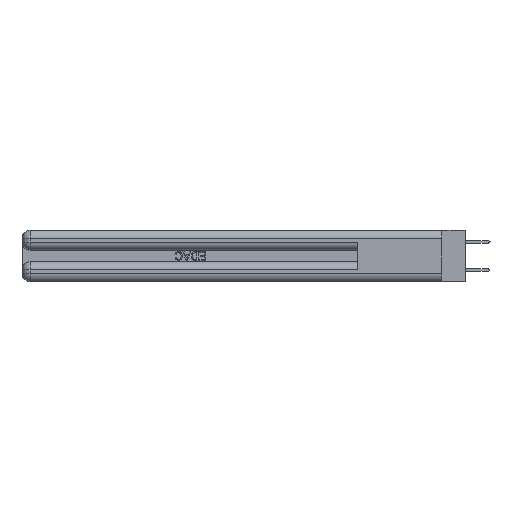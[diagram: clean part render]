
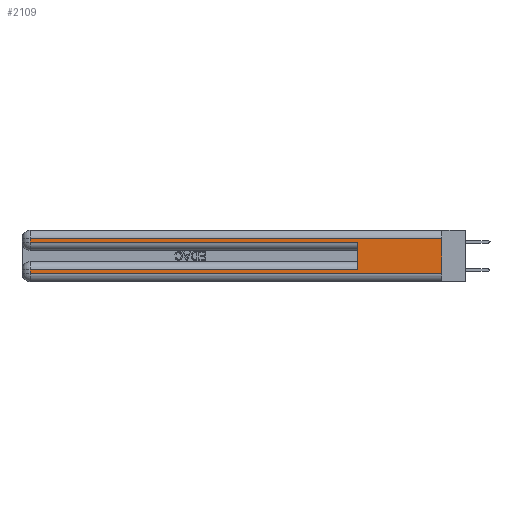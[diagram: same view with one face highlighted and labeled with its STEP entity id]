
A CAD part, left-side view. The second image highlights one B-rep face of the part: STEP entity #2109.
In plain terms, the highlighted planar face has unit normal (-1, 0, 0).
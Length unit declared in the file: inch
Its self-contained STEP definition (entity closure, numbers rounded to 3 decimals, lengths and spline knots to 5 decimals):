
#2109 = ADVANCED_FACE ( 'NONE', ( #13333 ), #38572, .F. ) ;
#3598 = CARTESIAN_POINT ( 'NONE',  ( 0., 0., 0.285 ) ) ;
#4173 = EDGE_CURVE ( 'NONE', #25780, #25477, #43261, .T. ) ;
#4603 = EDGE_CURVE ( 'NONE', #20547, #20723, #4740, .T. ) ;
#4740 = LINE ( 'NONE', #40680, #20423 ) ;
#5199 = LINE ( 'NONE', #25803, #18037 ) ;
#6324 = DIRECTION ( 'NONE',  ( 0., 0., -1. ) ) ;
#6469 = CARTESIAN_POINT ( 'NONE',  ( 0., 2.94, 0.06 ) ) ;
#7218 = VECTOR ( 'NONE', #45504, 39.37008 ) ;
#8037 = DIRECTION ( 'NONE',  ( 0., 1., 0. ) ) ;
#9441 = CARTESIAN_POINT ( 'NONE',  ( 0., 0.6, 0.145 ) ) ;
#11390 = AXIS2_PLACEMENT_3D ( 'NONE', #13796, #22963, #24110 ) ;
#11472 = DIRECTION ( 'NONE',  ( 0., -1., 0. ) ) ;
#12254 = LINE ( 'NONE', #9441, #7218 ) ;
#13333 = FACE_OUTER_BOUND ( 'NONE', #28089, .T. ) ;
#13796 = CARTESIAN_POINT ( 'NONE',  ( 0., 0., 0.37 ) ) ;
#14299 = LINE ( 'NONE', #3598, #29890 ) ;
#14329 = DIRECTION ( 'NONE',  ( 0., -1., 0. ) ) ;
#15424 = CARTESIAN_POINT ( 'NONE',  ( 0., 2.94, 0.285 ) ) ;
#16871 = EDGE_CURVE ( 'NONE', #22562, #25780, #21992, .T. ) ;
#17128 = DIRECTION ( 'NONE',  ( 0., 1., 0. ) ) ;
#17292 = CARTESIAN_POINT ( 'NONE',  ( 0., 0., 0.31 ) ) ;
#18037 = VECTOR ( 'NONE', #11472, 39.37008 ) ;
#19333 = DIRECTION ( 'NONE',  ( 0., 0., -1. ) ) ;
#20137 = CARTESIAN_POINT ( 'NONE',  ( 0., 0.6, 0.085 ) ) ;
#20184 = VERTEX_POINT ( 'NONE', #20137 ) ;
#20280 = ORIENTED_EDGE ( 'NONE', *, *, #42400, .T. ) ;
#20293 = VECTOR ( 'NONE', #17128, 39.37008 ) ;
#20423 = VECTOR ( 'NONE', #19333, 39.37008 ) ;
#20547 = VERTEX_POINT ( 'NONE', #36850 ) ;
#20723 = VERTEX_POINT ( 'NONE', #6469 ) ;
#21463 = VECTOR ( 'NONE', #8037, 39.37008 ) ;
#21992 = LINE ( 'NONE', #42281, #21463 ) ;
#22198 = CARTESIAN_POINT ( 'NONE',  ( 0., 0., 0.37 ) ) ;
#22562 = VERTEX_POINT ( 'NONE', #17292 ) ;
#22963 = DIRECTION ( 'NONE',  ( 1., 0., 0. ) ) ;
#23842 = VERTEX_POINT ( 'NONE', #34713 ) ;
#24110 = DIRECTION ( 'NONE',  ( 0., 0., -1. ) ) ;
#25477 = VERTEX_POINT ( 'NONE', #15424 ) ;
#25780 = VERTEX_POINT ( 'NONE', #31588 ) ;
#25803 = CARTESIAN_POINT ( 'NONE',  ( 0., 0., 0.06 ) ) ;
#26519 = EDGE_CURVE ( 'NONE', #22562, #23842, #26721, .T. ) ;
#26721 = LINE ( 'NONE', #22198, #40646 ) ;
#28089 = EDGE_LOOP ( 'NONE', ( #34887, #36094, #33146, #20280, #37297, #33915, #33321, #35977 ) ) ;
#28685 = CARTESIAN_POINT ( 'NONE',  ( 0., 2.94, 0.37 ) ) ;
#29672 = VERTEX_POINT ( 'NONE', #32117 ) ;
#29890 = VECTOR ( 'NONE', #14329, 39.37008 ) ;
#31278 = CARTESIAN_POINT ( 'NONE',  ( 0., 0., 0.085 ) ) ;
#31540 = EDGE_CURVE ( 'NONE', #20184, #29672, #12254, .T. ) ;
#31588 = CARTESIAN_POINT ( 'NONE',  ( 0., 2.94, 0.31 ) ) ;
#32117 = CARTESIAN_POINT ( 'NONE',  ( 0., 0.6, 0.285 ) ) ;
#33146 = ORIENTED_EDGE ( 'NONE', *, *, #4173, .T. ) ;
#33321 = ORIENTED_EDGE ( 'NONE', *, *, #4603, .T. ) ;
#33595 = LINE ( 'NONE', #31278, #20293 ) ;
#33915 = ORIENTED_EDGE ( 'NONE', *, *, #44064, .T. ) ;
#34713 = CARTESIAN_POINT ( 'NONE',  ( 0., 0., 0.06 ) ) ;
#34887 = ORIENTED_EDGE ( 'NONE', *, *, #26519, .F. ) ;
#35977 = ORIENTED_EDGE ( 'NONE', *, *, #37525, .T. ) ;
#36094 = ORIENTED_EDGE ( 'NONE', *, *, #16871, .T. ) ;
#36496 = VECTOR ( 'NONE', #44303, 39.37008 ) ;
#36850 = CARTESIAN_POINT ( 'NONE',  ( 0., 2.94, 0.085 ) ) ;
#37297 = ORIENTED_EDGE ( 'NONE', *, *, #31540, .F. ) ;
#37525 = EDGE_CURVE ( 'NONE', #20723, #23842, #5199, .T. ) ;
#38572 = PLANE ( 'NONE',  #11390 ) ;
#40646 = VECTOR ( 'NONE', #6324, 39.37008 ) ;
#40680 = CARTESIAN_POINT ( 'NONE',  ( 0., 2.94, 0.37 ) ) ;
#42281 = CARTESIAN_POINT ( 'NONE',  ( 0., 0., 0.31 ) ) ;
#42400 = EDGE_CURVE ( 'NONE', #25477, #29672, #14299, .T. ) ;
#43261 = LINE ( 'NONE', #28685, #36496 ) ;
#44064 = EDGE_CURVE ( 'NONE', #20184, #20547, #33595, .T. ) ;
#44303 = DIRECTION ( 'NONE',  ( 0., 0., -1. ) ) ;
#45504 = DIRECTION ( 'NONE',  ( 0., 0., 1. ) ) ;
